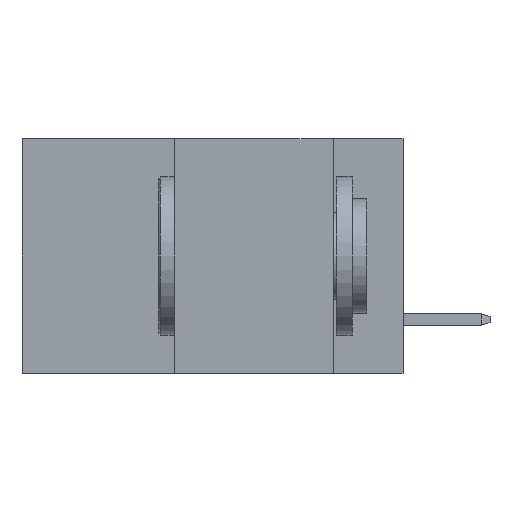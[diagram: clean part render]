
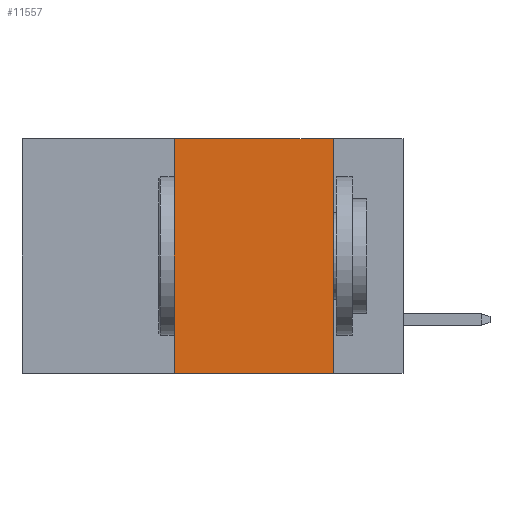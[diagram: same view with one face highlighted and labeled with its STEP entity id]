
A CAD part, left-side view. The second image highlights one B-rep face of the part: STEP entity #11557.
In plain terms, the highlighted planar face has unit normal (-1, 0, 0).
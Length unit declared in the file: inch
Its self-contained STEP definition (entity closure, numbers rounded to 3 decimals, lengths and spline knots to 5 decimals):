
#94 = VERTEX_POINT ( 'NONE', #7727 ) ;
#739 = AXIS2_PLACEMENT_3D ( 'NONE', #7696, #12381, #2454 ) ;
#1622 = CARTESIAN_POINT ( 'NONE',  ( 0., 0.11, 0. ) ) ;
#1967 = DIRECTION ( 'NONE',  ( 0., 0., -1. ) ) ;
#2454 = DIRECTION ( 'NONE',  ( 0., 0., -1. ) ) ;
#2616 = CARTESIAN_POINT ( 'NONE',  ( 0., 0.6, 0. ) ) ;
#2794 = CARTESIAN_POINT ( 'NONE',  ( 0., 0.6, -0.37 ) ) ;
#3266 = VERTEX_POINT ( 'NONE', #14086 ) ;
#3511 = CARTESIAN_POINT ( 'NONE',  ( 0., 0.11, 0. ) ) ;
#4234 = ORIENTED_EDGE ( 'NONE', *, *, #6806, .F. ) ;
#4549 = ORIENTED_EDGE ( 'NONE', *, *, #14125, .F. ) ;
#5012 = LINE ( 'NONE', #2616, #5260 ) ;
#5197 = VECTOR ( 'NONE', #12897, 39.37008 ) ;
#5260 = VECTOR ( 'NONE', #6011, 39.37008 ) ;
#5327 = VERTEX_POINT ( 'NONE', #1622 ) ;
#5456 = VECTOR ( 'NONE', #8941, 39.37008 ) ;
#5630 = ORIENTED_EDGE ( 'NONE', *, *, #6159, .F. ) ;
#5942 = CARTESIAN_POINT ( 'NONE',  ( 0., 0.36, 0. ) ) ;
#6011 = DIRECTION ( 'NONE',  ( 0., -1., 0. ) ) ;
#6159 = EDGE_CURVE ( 'NONE', #9063, #5327, #5012, .T. ) ;
#6476 = FACE_OUTER_BOUND ( 'NONE', #6695, .T. ) ;
#6513 = VECTOR ( 'NONE', #1967, 39.37008 ) ;
#6695 = EDGE_LOOP ( 'NONE', ( #4234, #5630, #4549, #9941 ) ) ;
#6806 = EDGE_CURVE ( 'NONE', #5327, #3266, #10340, .T. ) ;
#7696 = CARTESIAN_POINT ( 'NONE',  ( 0., 0.6, 0. ) ) ;
#7727 = CARTESIAN_POINT ( 'NONE',  ( 0., 0.36, -0.37 ) ) ;
#8442 = LINE ( 'NONE', #13125, #5197 ) ;
#8941 = DIRECTION ( 'NONE',  ( 0., -1., 0. ) ) ;
#9063 = VERTEX_POINT ( 'NONE', #5942 ) ;
#9941 = ORIENTED_EDGE ( 'NONE', *, *, #12778, .T. ) ;
#10071 = PLANE ( 'NONE',  #739 ) ;
#10340 = LINE ( 'NONE', #3511, #6513 ) ;
#11557 = ADVANCED_FACE ( 'NONE', ( #6476 ), #10071, .F. ) ;
#12381 = DIRECTION ( 'NONE',  ( 1., 0., 0. ) ) ;
#12778 = EDGE_CURVE ( 'NONE', #94, #3266, #13470, .T. ) ;
#12897 = DIRECTION ( 'NONE',  ( 0., 0., 1. ) ) ;
#13125 = CARTESIAN_POINT ( 'NONE',  ( 0., 0.36, 0. ) ) ;
#13470 = LINE ( 'NONE', #2794, #5456 ) ;
#14086 = CARTESIAN_POINT ( 'NONE',  ( 0., 0.11, -0.37 ) ) ;
#14125 = EDGE_CURVE ( 'NONE', #94, #9063, #8442, .T. ) ;
